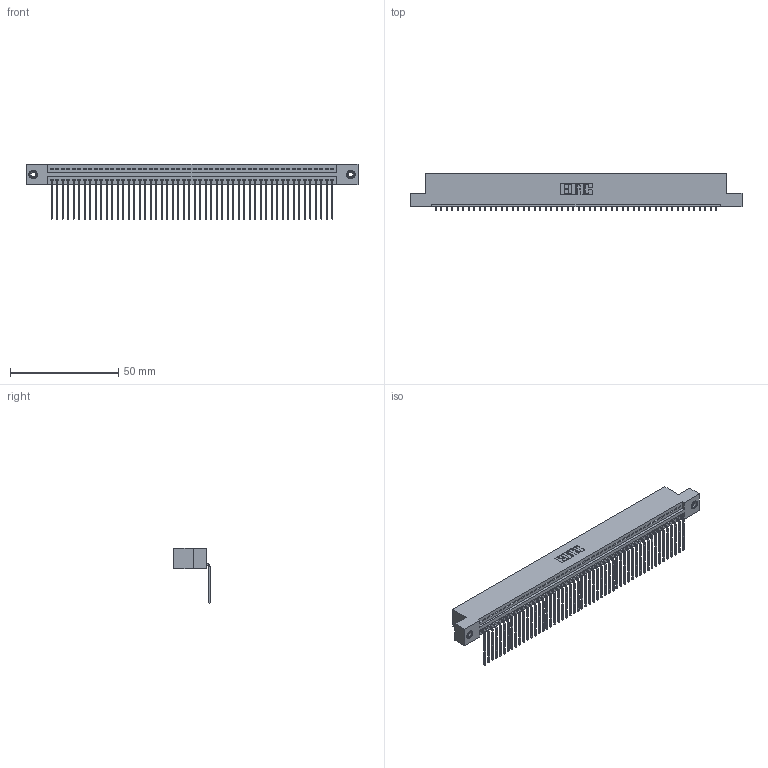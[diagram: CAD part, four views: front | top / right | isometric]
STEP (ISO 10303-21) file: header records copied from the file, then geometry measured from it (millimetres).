
FILE_DESCRIPTION (( 'STEP AP203' ), '1' );
FILE_NAME ('395-052-559-108.STEP', '2018-11-21T01:57:45', ( '' ), ( '' ), 'SwSTEP 2.0', 'SolidWorks 2016', '' );
FILE_SCHEMA (( 'CONFIG_CONTROL_DESIGN' ));
Length unit declared in the file: inch
Products named in the file (4): 345 Part_Flush Mounting Lugs - 0.156 Dia-TI; 345-292-001_558 559 Tail - 1; 345-250-001_345-250-003-102; 395-052-559-108
Assembly tree (55 placements, depth 2):
  395-052-559-108
    345 Part_Flush Mounting Lugs - 0.156 Dia-TI
    345-292-001_558 559 Tail - 1  x52
    345-250-001_345-250-003-102  x2
Bounding box: 153.29 x 16.75 x 25.53 mm (x, y, z)
Volume: 14808.2 mm3; surface area: 20851.9 mm2
Topology: 55 solids, 55 shells, 3306 faces, 9941 edges, 6550 vertices
Faces by surface type: plane 2296, cylinder 994, cone 12, torus 4
Entity records: 39060 total; most frequent: CARTESIAN_POINT 6747, ORIENTED_EDGE 6726, DIRECTION 5905, EDGE_CURVE 3363, LINE 3003, VECTOR 3003, VERTEX_POINT 2236, AXIS2_PLACEMENT_3D 1451
